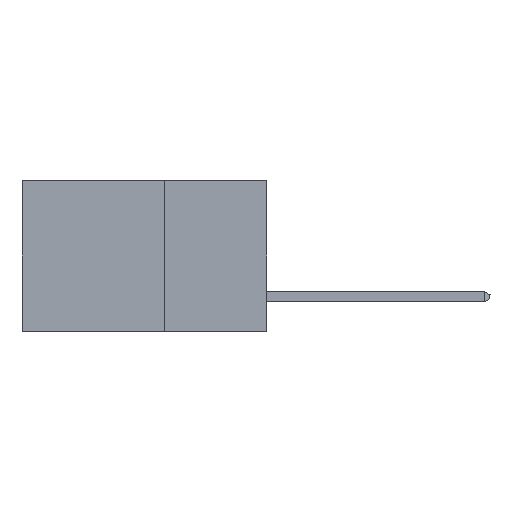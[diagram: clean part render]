
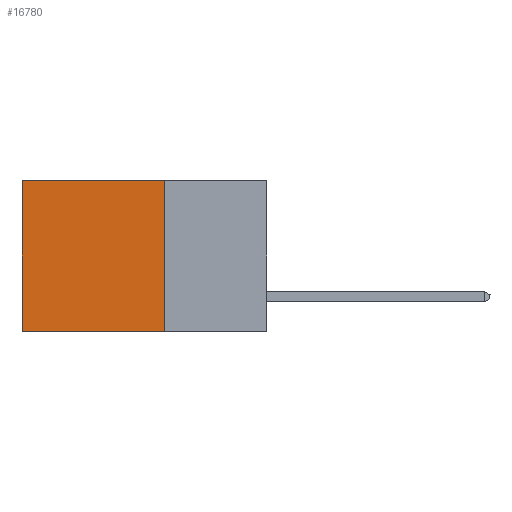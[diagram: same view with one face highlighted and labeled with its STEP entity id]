
A CAD part, left-side view. The second image highlights one B-rep face of the part: STEP entity #16780.
In plain terms, the highlighted planar face has unit normal (-1, 0, 0).
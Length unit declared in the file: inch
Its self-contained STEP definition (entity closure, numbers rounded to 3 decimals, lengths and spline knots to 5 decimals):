
#39 = CARTESIAN_POINT ( 'NONE',  ( 0.2875, 0.6, -0.37 ) ) ;
#1007 = VECTOR ( 'NONE', #8642, 39.37008 ) ;
#2440 = EDGE_CURVE ( 'NONE', #10364, #14462, #18164, .T. ) ;
#4311 = VECTOR ( 'NONE', #7599, 39.37008 ) ;
#4996 = FACE_OUTER_BOUND ( 'NONE', #23397, .T. ) ;
#5134 = PLANE ( 'NONE',  #6892 ) ;
#6098 = CARTESIAN_POINT ( 'NONE',  ( 0.2875, 0.25, -0.37 ) ) ;
#6203 = LINE ( 'NONE', #14961, #1007 ) ;
#6618 = ORIENTED_EDGE ( 'NONE', *, *, #19915, .F. ) ;
#6892 = AXIS2_PLACEMENT_3D ( 'NONE', #22635, #9164, #20507 ) ;
#7456 = CARTESIAN_POINT ( 'NONE',  ( 0.2875, 0.25, 0. ) ) ;
#7599 = DIRECTION ( 'NONE',  ( 0., 0., -1. ) ) ;
#7737 = LINE ( 'NONE', #7456, #4311 ) ;
#8307 = EDGE_CURVE ( 'NONE', #10364, #25448, #7737, .T. ) ;
#8642 = DIRECTION ( 'NONE',  ( 0., 0., -1. ) ) ;
#9164 = DIRECTION ( 'NONE',  ( 1., 0., 0. ) ) ;
#10364 = VERTEX_POINT ( 'NONE', #26336 ) ;
#11544 = CARTESIAN_POINT ( 'NONE',  ( 0.2875, 0.6, 0. ) ) ;
#12144 = ORIENTED_EDGE ( 'NONE', *, *, #20449, .T. ) ;
#12500 = ORIENTED_EDGE ( 'NONE', *, *, #8307, .F. ) ;
#13541 = VERTEX_POINT ( 'NONE', #39 ) ;
#14462 = VERTEX_POINT ( 'NONE', #11544 ) ;
#14961 = CARTESIAN_POINT ( 'NONE',  ( 0.2875, 0.6, 0. ) ) ;
#16443 = DIRECTION ( 'NONE',  ( 0., 1., 0. ) ) ;
#16471 = VECTOR ( 'NONE', #26918, 39.37008 ) ;
#16780 = ADVANCED_FACE ( 'NONE', ( #4996 ), #5134, .F. ) ;
#18164 = LINE ( 'NONE', #27056, #16471 ) ;
#18452 = CARTESIAN_POINT ( 'NONE',  ( 0.2875, 0.25, -0.37 ) ) ;
#18517 = ORIENTED_EDGE ( 'NONE', *, *, #2440, .T. ) ;
#19915 = EDGE_CURVE ( 'NONE', #25448, #13541, #25329, .T. ) ;
#20449 = EDGE_CURVE ( 'NONE', #14462, #13541, #6203, .T. ) ;
#20507 = DIRECTION ( 'NONE',  ( 0., 0., -1. ) ) ;
#21130 = VECTOR ( 'NONE', #16443, 39.37008 ) ;
#22635 = CARTESIAN_POINT ( 'NONE',  ( 0.2875, 0.25, 0. ) ) ;
#23397 = EDGE_LOOP ( 'NONE', ( #12144, #6618, #12500, #18517 ) ) ;
#25329 = LINE ( 'NONE', #18452, #21130 ) ;
#25448 = VERTEX_POINT ( 'NONE', #6098 ) ;
#26336 = CARTESIAN_POINT ( 'NONE',  ( 0.2875, 0.25, 0. ) ) ;
#26918 = DIRECTION ( 'NONE',  ( 0., 1., 0. ) ) ;
#27056 = CARTESIAN_POINT ( 'NONE',  ( 0.2875, 0.25, 0. ) ) ;
